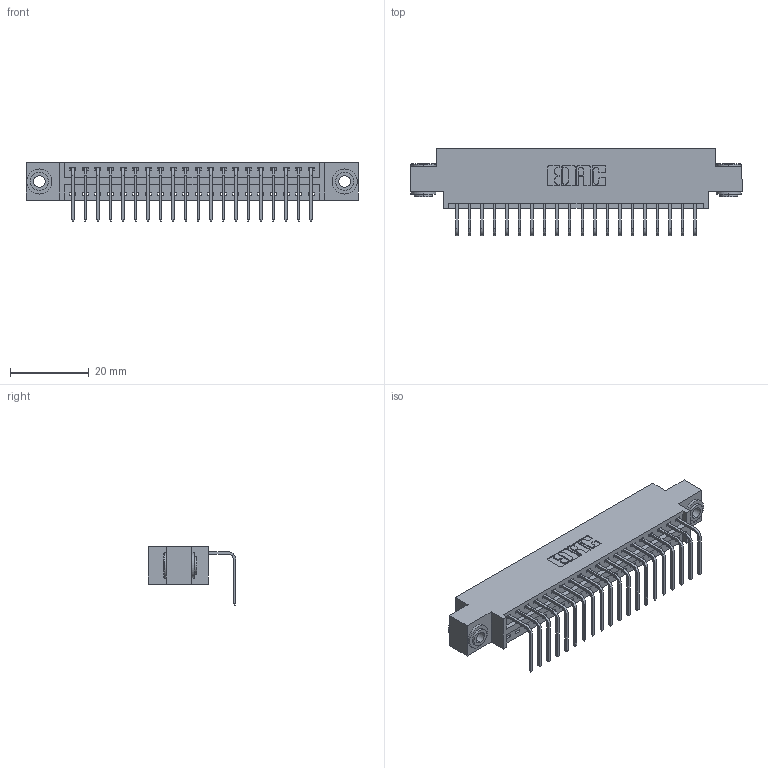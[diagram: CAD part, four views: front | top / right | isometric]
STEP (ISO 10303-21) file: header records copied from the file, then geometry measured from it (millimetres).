
FILE_DESCRIPTION (( 'STEP AP203' ), '1' );
FILE_NAME ('346-020-558-603.STEP', '2022-05-05T17:09:34', ( '' ), ( '' ), 'SwSTEP 2.0', 'SolidWorks 2020', '' );
FILE_SCHEMA (( 'CONFIG_CONTROL_DESIGN' ));
Length unit declared in the file: inch
Products named in the file (4): 345-292-001_558 Tail - 2; 346 Part_0.170 Offset - 0.156 Dia-TH; 346-020-558-603; 345-250-002_345-250-002-102
Assembly tree (23 placements, depth 2):
  346-020-558-603
    346 Part_0.170 Offset - 0.156 Dia-TH
    345-292-001_558 Tail - 2  x20
    345-250-002_345-250-002-102  x2
Bounding box: 84.07 x 22.16 x 14.73 mm (x, y, z)
Volume: 7809.5 mm3; surface area: 10332.8 mm2
Topology: 23 solids, 23 shells, 1378 faces, 4093 edges, 2698 vertices
Faces by surface type: plane 944, cylinder 426, cone 8
Entity records: 16656 total; most frequent: CARTESIAN_POINT 2845, ORIENTED_EDGE 2790, DIRECTION 2565, EDGE_CURVE 1395, VECTOR 1159, LINE 1159, VERTEX_POINT 926, AXIS2_PLACEMENT_3D 703
